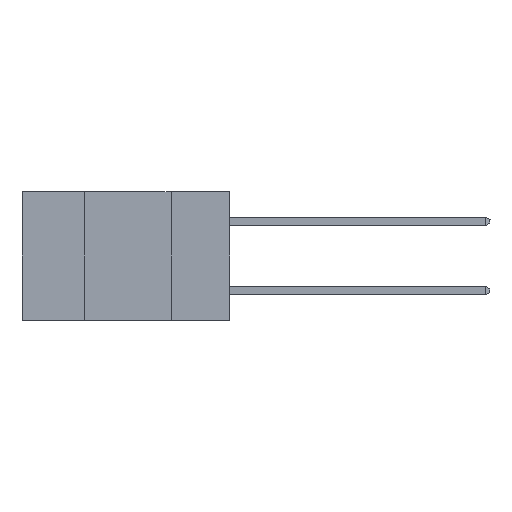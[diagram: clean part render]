
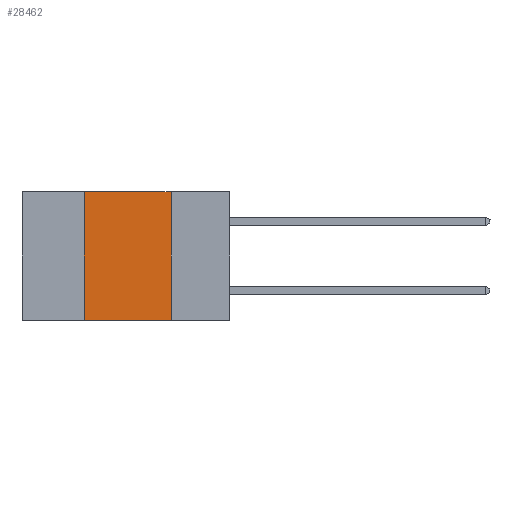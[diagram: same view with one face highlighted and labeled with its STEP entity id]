
A CAD part, left-side view. The second image highlights one B-rep face of the part: STEP entity #28462.
In plain terms, the highlighted planar face has unit normal (-1, 0, 0).
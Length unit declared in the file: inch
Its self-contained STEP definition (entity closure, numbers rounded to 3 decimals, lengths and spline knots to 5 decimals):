
#850 = CARTESIAN_POINT ( 'NONE',  ( 0., 0.17, 0. ) ) ;
#1348 = ORIENTED_EDGE ( 'NONE', *, *, #17895, .T. ) ;
#2841 = EDGE_CURVE ( 'NONE', #6024, #6310, #23815, .T. ) ;
#2855 = DIRECTION ( 'NONE',  ( 1., 0., 0. ) ) ;
#3179 = CARTESIAN_POINT ( 'NONE',  ( 0., 0.6, 0. ) ) ;
#4947 = VERTEX_POINT ( 'NONE', #15310 ) ;
#5504 = DIRECTION ( 'NONE',  ( 0., 0., 1. ) ) ;
#5648 = DIRECTION ( 'NONE',  ( 0., 0., -1. ) ) ;
#6024 = VERTEX_POINT ( 'NONE', #18135 ) ;
#6310 = VERTEX_POINT ( 'NONE', #29555 ) ;
#6902 = DIRECTION ( 'NONE',  ( 0., -1., 0. ) ) ;
#7443 = LINE ( 'NONE', #850, #24195 ) ;
#8233 = CARTESIAN_POINT ( 'NONE',  ( 0., 0.42, 0. ) ) ;
#9932 = VECTOR ( 'NONE', #20112, 39.37008 ) ;
#10619 = FACE_OUTER_BOUND ( 'NONE', #22910, .T. ) ;
#11786 = CARTESIAN_POINT ( 'NONE',  ( 0., 0.6, 0. ) ) ;
#13854 = EDGE_CURVE ( 'NONE', #6310, #18725, #7443, .T. ) ;
#14040 = LINE ( 'NONE', #15625, #9932 ) ;
#14250 = EDGE_CURVE ( 'NONE', #4947, #6024, #28620, .T. ) ;
#15310 = CARTESIAN_POINT ( 'NONE',  ( 0., 0.42, -0.37 ) ) ;
#15625 = CARTESIAN_POINT ( 'NONE',  ( 0., 0.6, -0.37 ) ) ;
#17379 = ORIENTED_EDGE ( 'NONE', *, *, #14250, .F. ) ;
#17895 = EDGE_CURVE ( 'NONE', #4947, #18725, #14040, .T. ) ;
#18135 = CARTESIAN_POINT ( 'NONE',  ( 0., 0.42, 0. ) ) ;
#18204 = VECTOR ( 'NONE', #5504, 39.37008 ) ;
#18725 = VERTEX_POINT ( 'NONE', #26130 ) ;
#19223 = ORIENTED_EDGE ( 'NONE', *, *, #13854, .F. ) ;
#20112 = DIRECTION ( 'NONE',  ( 0., -1., 0. ) ) ;
#21544 = VECTOR ( 'NONE', #6902, 39.37008 ) ;
#22358 = ORIENTED_EDGE ( 'NONE', *, *, #2841, .F. ) ;
#22910 = EDGE_LOOP ( 'NONE', ( #19223, #22358, #17379, #1348 ) ) ;
#23815 = LINE ( 'NONE', #11786, #21544 ) ;
#24195 = VECTOR ( 'NONE', #5648, 39.37008 ) ;
#24424 = PLANE ( 'NONE',  #29627 ) ;
#24615 = DIRECTION ( 'NONE',  ( 0., 0., -1. ) ) ;
#26130 = CARTESIAN_POINT ( 'NONE',  ( 0., 0.17, -0.37 ) ) ;
#28462 = ADVANCED_FACE ( 'NONE', ( #10619 ), #24424, .F. ) ;
#28620 = LINE ( 'NONE', #8233, #18204 ) ;
#29555 = CARTESIAN_POINT ( 'NONE',  ( 0., 0.17, 0. ) ) ;
#29627 = AXIS2_PLACEMENT_3D ( 'NONE', #3179, #2855, #24615 ) ;
